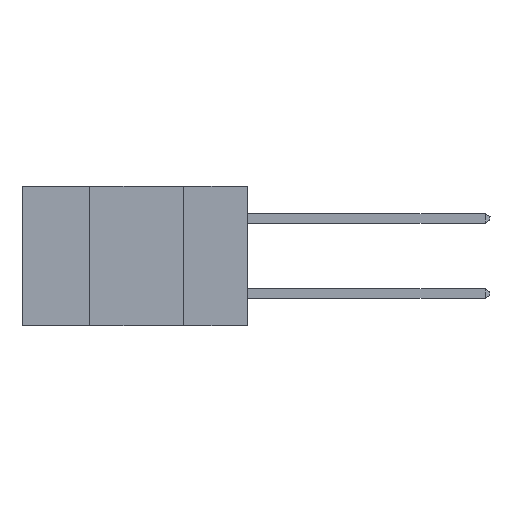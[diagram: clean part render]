
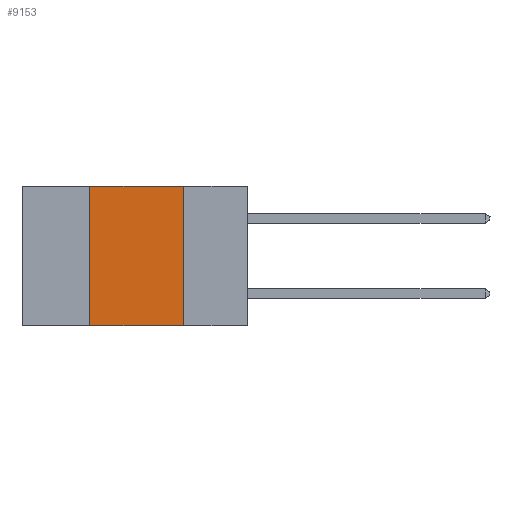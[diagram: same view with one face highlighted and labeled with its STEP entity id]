
A CAD part, left-side view. The second image highlights one B-rep face of the part: STEP entity #9153.
In plain terms, the highlighted planar face has unit normal (-1, 0, 0).
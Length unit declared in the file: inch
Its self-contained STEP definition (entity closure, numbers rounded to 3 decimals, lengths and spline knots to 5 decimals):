
#459 = CARTESIAN_POINT ( 'NONE',  ( 0., 0.6, 0. ) ) ;
#485 = EDGE_CURVE ( 'NONE', #7973, #622, #17957, .T. ) ;
#587 = CARTESIAN_POINT ( 'NONE',  ( 0., 0.42, -0.37 ) ) ;
#622 = VERTEX_POINT ( 'NONE', #10655 ) ;
#963 = AXIS2_PLACEMENT_3D ( 'NONE', #459, #14750, #16424 ) ;
#1086 = ORIENTED_EDGE ( 'NONE', *, *, #1140, .T. ) ;
#1140 = EDGE_CURVE ( 'NONE', #7973, #13576, #16615, .T. ) ;
#2159 = CARTESIAN_POINT ( 'NONE',  ( 0., 0.6, 0. ) ) ;
#2350 = DIRECTION ( 'NONE',  ( 0., -1., 0. ) ) ;
#3003 = ORIENTED_EDGE ( 'NONE', *, *, #485, .F. ) ;
#3649 = PLANE ( 'NONE',  #963 ) ;
#3842 = CARTESIAN_POINT ( 'NONE',  ( 0., 0.6, -0.37 ) ) ;
#4981 = CARTESIAN_POINT ( 'NONE',  ( 0., 0.17, -0.37 ) ) ;
#5186 = CARTESIAN_POINT ( 'NONE',  ( 0., 0.17, 0. ) ) ;
#7711 = FACE_OUTER_BOUND ( 'NONE', #17185, .T. ) ;
#7843 = DIRECTION ( 'NONE',  ( 0., 0., 1. ) ) ;
#7973 = VERTEX_POINT ( 'NONE', #9837 ) ;
#8100 = DIRECTION ( 'NONE',  ( 0., -1., 0. ) ) ;
#8335 = VECTOR ( 'NONE', #7843, 39.37008 ) ;
#8420 = VECTOR ( 'NONE', #8100, 39.37008 ) ;
#9153 = ADVANCED_FACE ( 'NONE', ( #7711 ), #3649, .F. ) ;
#9830 = VERTEX_POINT ( 'NONE', #5186 ) ;
#9837 = CARTESIAN_POINT ( 'NONE',  ( 0., 0.42, -0.37 ) ) ;
#10072 = EDGE_CURVE ( 'NONE', #622, #9830, #13670, .T. ) ;
#10655 = CARTESIAN_POINT ( 'NONE',  ( 0., 0.42, 0. ) ) ;
#11155 = ORIENTED_EDGE ( 'NONE', *, *, #10072, .F. ) ;
#11417 = VECTOR ( 'NONE', #17671, 39.37008 ) ;
#12055 = LINE ( 'NONE', #16346, #11417 ) ;
#12607 = VECTOR ( 'NONE', #2350, 39.37008 ) ;
#13576 = VERTEX_POINT ( 'NONE', #4981 ) ;
#13670 = LINE ( 'NONE', #2159, #12607 ) ;
#14750 = DIRECTION ( 'NONE',  ( 1., 0., 0. ) ) ;
#15411 = EDGE_CURVE ( 'NONE', #9830, #13576, #12055, .T. ) ;
#16346 = CARTESIAN_POINT ( 'NONE',  ( 0., 0.17, -0.37 ) ) ;
#16424 = DIRECTION ( 'NONE',  ( 0., 0., -1. ) ) ;
#16615 = LINE ( 'NONE', #3842, #8420 ) ;
#16951 = ORIENTED_EDGE ( 'NONE', *, *, #15411, .F. ) ;
#17185 = EDGE_LOOP ( 'NONE', ( #16951, #11155, #3003, #1086 ) ) ;
#17671 = DIRECTION ( 'NONE',  ( 0., 0., -1. ) ) ;
#17957 = LINE ( 'NONE', #587, #8335 ) ;
